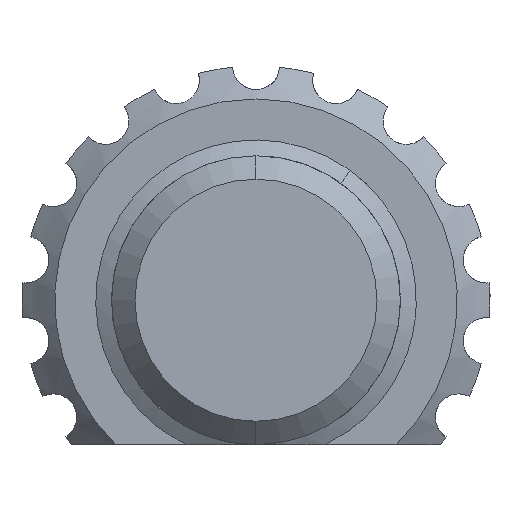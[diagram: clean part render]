
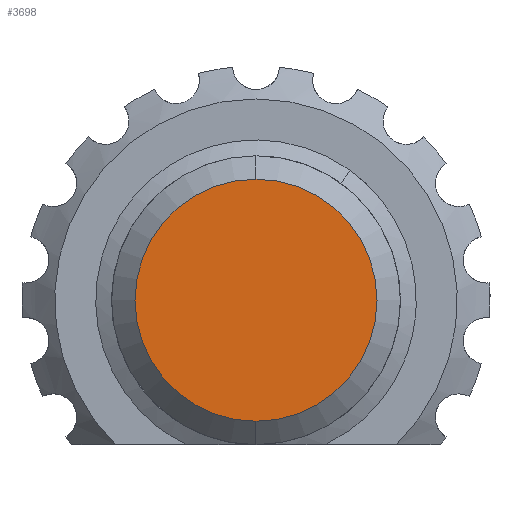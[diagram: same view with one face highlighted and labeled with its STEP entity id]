
A CAD part, left-side view. The second image highlights one B-rep face of the part: STEP entity #3698.
In plain terms, the highlighted planar face has unit normal (-1, 0, 0).
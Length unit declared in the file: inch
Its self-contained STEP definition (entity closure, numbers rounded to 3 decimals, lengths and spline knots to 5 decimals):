
#100 = DIRECTION ( 'NONE',  ( 0., 0., -1. ) ) ;
#123 = DIRECTION ( 'NONE',  ( -1., 0., 0. ) ) ;
#649 = CARTESIAN_POINT ( 'NONE',  ( -0.5675, 0.5675, 0.04883 ) ) ;
#897 = CARTESIAN_POINT ( 'NONE',  ( -0.5675, 0.5675, -0.08042 ) ) ;
#1440 = VERTEX_POINT ( 'NONE', #649 ) ;
#2181 = EDGE_LOOP ( 'NONE', ( #6501, #5478 ) ) ;
#3663 = DIRECTION ( 'NONE',  ( -1., 0., 0. ) ) ;
#3674 = PLANE ( 'NONE',  #8774 ) ;
#3698 = ADVANCED_FACE ( 'NONE', ( #6252 ), #3674, .F. ) ;
#4023 = CIRCLE ( 'NONE', #9368, 0.12925 ) ;
#4360 = EDGE_CURVE ( 'NONE', #1440, #9208, #4023, .T. ) ;
#4414 = DIRECTION ( 'NONE',  ( 0., 0., -1. ) ) ;
#4696 = CARTESIAN_POINT ( 'NONE',  ( -0.5675, 0.5675, -0.20967 ) ) ;
#5405 = DIRECTION ( 'NONE',  ( 0., 0., -1. ) ) ;
#5478 = ORIENTED_EDGE ( 'NONE', *, *, #4360, .T. ) ;
#6249 = AXIS2_PLACEMENT_3D ( 'NONE', #9708, #123, #4414 ) ;
#6252 = FACE_OUTER_BOUND ( 'NONE', #2181, .T. ) ;
#6501 = ORIENTED_EDGE ( 'NONE', *, *, #10645, .T. ) ;
#7665 = CIRCLE ( 'NONE', #6249, 0.12925 ) ;
#7916 = DIRECTION ( 'NONE',  ( 1., 0., 0. ) ) ;
#8774 = AXIS2_PLACEMENT_3D ( 'NONE', #10603, #7916, #5405 ) ;
#9208 = VERTEX_POINT ( 'NONE', #4696 ) ;
#9368 = AXIS2_PLACEMENT_3D ( 'NONE', #897, #3663, #100 ) ;
#9708 = CARTESIAN_POINT ( 'NONE',  ( -0.5675, 0.5675, -0.08042 ) ) ;
#10603 = CARTESIAN_POINT ( 'NONE',  ( -0.5675, 0.5675, -0.08042 ) ) ;
#10645 = EDGE_CURVE ( 'NONE', #9208, #1440, #7665, .T. ) ;
